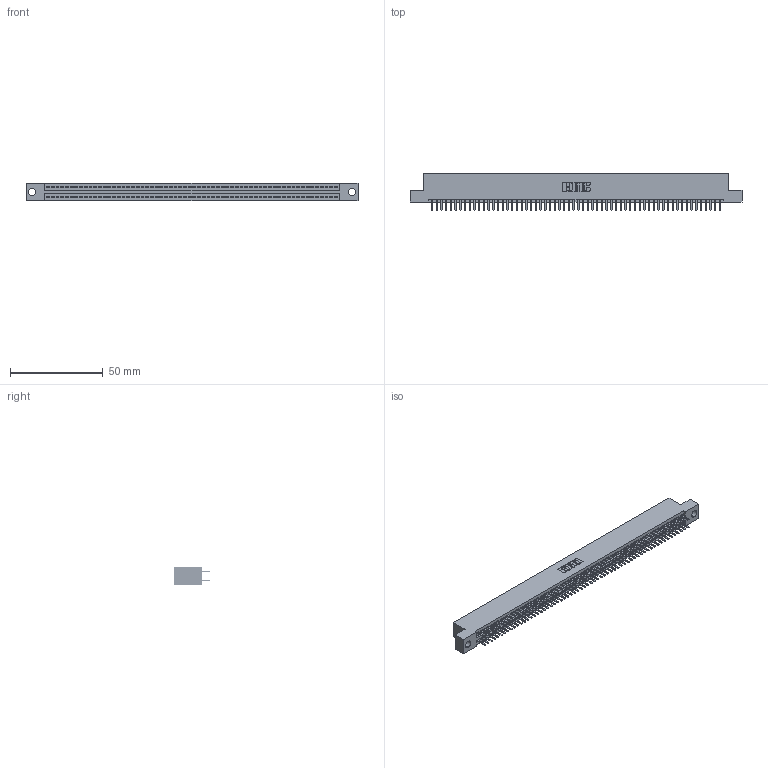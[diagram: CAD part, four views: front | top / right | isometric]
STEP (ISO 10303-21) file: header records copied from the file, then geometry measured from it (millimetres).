
FILE_DESCRIPTION (( 'STEP AP203' ), '1' );
FILE_NAME ('395-124-520-204.STEP', '2018-12-03T21:32:35', ( '' ), ( '' ), 'SwSTEP 2.0', 'SolidWorks 2016', '' );
FILE_SCHEMA (( 'CONFIG_CONTROL_DESIGN' ));
Length unit declared in the file: inch
Products named in the file (3): 345 Part_Flush Mounting Lugs - 0.156 Dia-TH; 395-124-520-204; 345-292-001_345-293-120
Assembly tree (125 placements, depth 2):
  395-124-520-204
    345 Part_Flush Mounting Lugs - 0.156 Dia-TH
    345-292-001_345-293-120  x124
Bounding box: 178.69 x 19.68 x 9.4 mm (x, y, z)
Volume: 17401.3 mm3; surface area: 25808.7 mm2
Topology: 125 solids, 125 shells, 6822 faces, 19809 edges, 12874 vertices
Faces by surface type: plane 4420, cylinder 2402
Entity records: 46071 total; most frequent: CARTESIAN_POINT 7716, ORIENTED_EDGE 7638, DIRECTION 6767, EDGE_CURVE 3819, VECTOR 3435, LINE 3435, VERTEX_POINT 2542, AXIS2_PLACEMENT_3D 1666
